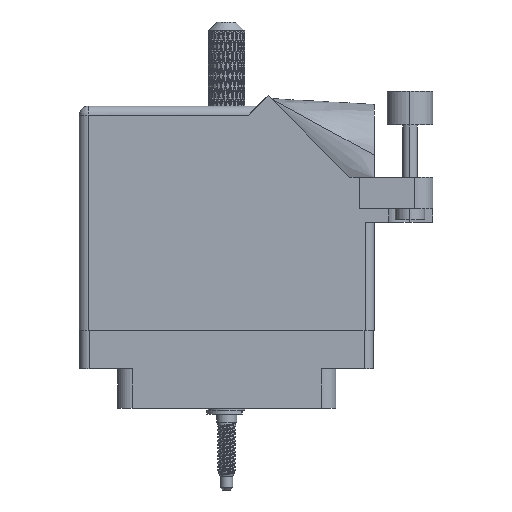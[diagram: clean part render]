
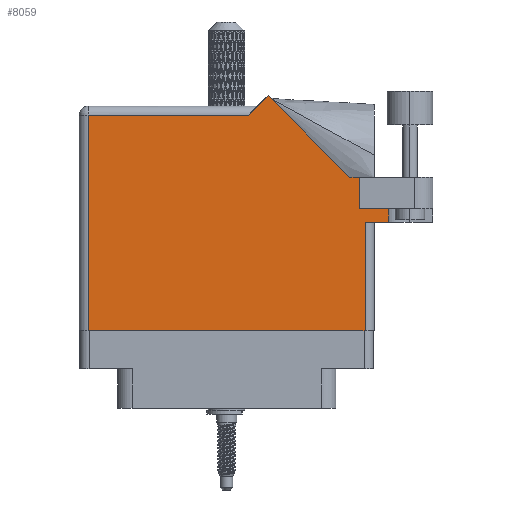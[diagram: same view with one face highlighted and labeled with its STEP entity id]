
A CAD part, front view. The second image highlights one B-rep face of the part: STEP entity #8059.
In plain terms, the highlighted face is planar.
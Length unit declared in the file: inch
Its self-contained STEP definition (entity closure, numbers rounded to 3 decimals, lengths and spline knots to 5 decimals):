
#267 = ORIENTED_EDGE ( 'NONE', *, *, #21707, .T. ) ;
#1807 = VECTOR ( 'NONE', #85075, 39.37008 ) ;
#2405 = VECTOR ( 'NONE', #69636, 39.37008 ) ;
#3095 = LINE ( 'NONE', #85515, #6949 ) ;
#5131 = CARTESIAN_POINT ( 'NONE',  ( 1.91, 0.831, 0. ) ) ;
#5653 = LINE ( 'NONE', #69418, #1807 ) ;
#6949 = VECTOR ( 'NONE', #50092, 39.37008 ) ;
#8059 = ADVANCED_FACE ( 'NONE', ( #53027 ), #77841, .F. ) ;
#8136 = DIRECTION ( 'NONE',  ( -1., 0., 0. ) ) ;
#8441 = DIRECTION ( 'NONE',  ( 0., 1., 0. ) ) ;
#9193 = LINE ( 'NONE', #20902, #78951 ) ;
#15080 = VERTEX_POINT ( 'NONE', #63916 ) ;
#15807 = CARTESIAN_POINT ( 'NONE',  ( 1.91, 0.831, 0. ) ) ;
#18346 = VERTEX_POINT ( 'NONE', #102619 ) ;
#19909 = VECTOR ( 'NONE', #8136, 39.37008 ) ;
#20902 = CARTESIAN_POINT ( 'NONE',  ( 0.062, 0., 0. ) ) ;
#21707 = EDGE_CURVE ( 'NONE', #97203, #96389, #76331, .T. ) ;
#24093 = CARTESIAN_POINT ( 'NONE',  ( 0., 1.468, 0. ) ) ;
#25519 = CARTESIAN_POINT ( 'NONE',  ( 2.1115, 0.737, 0. ) ) ;
#25620 = LINE ( 'NONE', #51140, #97981 ) ;
#27400 = EDGE_CURVE ( 'NONE', #18346, #99233, #84710, .T. ) ;
#27518 = EDGE_LOOP ( 'NONE', ( #94207, #48665, #95513, #96417, #34351, #267, #37238, #93862, #74592, #65399, #103088 ) ) ;
#27914 = AXIS2_PLACEMENT_3D ( 'NONE', #68934, #44972, #101667 ) ;
#28590 = CARTESIAN_POINT ( 'NONE',  ( 0.062, 0., 0. ) ) ;
#29988 = DIRECTION ( 'NONE',  ( 1., 0., 0. ) ) ;
#31210 = DIRECTION ( 'NONE',  ( 1., 0., 0. ) ) ;
#33255 = DIRECTION ( 'NONE',  ( -0.707, 0.707, 0. ) ) ;
#33606 = VERTEX_POINT ( 'NONE', #64223 ) ;
#34351 = ORIENTED_EDGE ( 'NONE', *, *, #74058, .F. ) ;
#37238 = ORIENTED_EDGE ( 'NONE', *, *, #104249, .T. ) ;
#38923 = LINE ( 'NONE', #98473, #65390 ) ;
#39635 = DIRECTION ( 'NONE',  ( 0., 1., 0. ) ) ;
#40151 = VECTOR ( 'NONE', #31210, 39.37008 ) ;
#41681 = VERTEX_POINT ( 'NONE', #93233 ) ;
#43035 = DIRECTION ( 'NONE',  ( 1., 0., 0. ) ) ;
#44609 = CARTESIAN_POINT ( 'NONE',  ( 2.1115, 0.831, 0. ) ) ;
#44972 = DIRECTION ( 'NONE',  ( 0., 0., -1. ) ) ;
#45186 = EDGE_CURVE ( 'NONE', #15080, #100135, #9193, .T. ) ;
#48665 = ORIENTED_EDGE ( 'NONE', *, *, #88799, .T. ) ;
#50092 = DIRECTION ( 'NONE',  ( -1., 0., 0. ) ) ;
#51140 = CARTESIAN_POINT ( 'NONE',  ( 2.01, 0.737, 0. ) ) ;
#53027 = FACE_OUTER_BOUND ( 'NONE', #27518, .T. ) ;
#53054 = EDGE_CURVE ( 'NONE', #41681, #79997, #25620, .T. ) ;
#53318 = CARTESIAN_POINT ( 'NONE',  ( 0., 0., 0. ) ) ;
#56301 = CARTESIAN_POINT ( 'NONE',  ( 1.948, 0.737, 0. ) ) ;
#57269 = VERTEX_POINT ( 'NONE', #44609 ) ;
#61670 = LINE ( 'NONE', #104939, #40151 ) ;
#61741 = EDGE_CURVE ( 'NONE', #100135, #33606, #100624, .T. ) ;
#63916 = CARTESIAN_POINT ( 'NONE',  ( 0.062, 1.468, 0. ) ) ;
#64223 = CARTESIAN_POINT ( 'NONE',  ( 1.948, 0., 0. ) ) ;
#65000 = VECTOR ( 'NONE', #39635, 39.37008 ) ;
#65390 = VECTOR ( 'NONE', #33255, 39.37008 ) ;
#65399 = ORIENTED_EDGE ( 'NONE', *, *, #86586, .T. ) ;
#68362 = DIRECTION ( 'NONE',  ( 0., -1., 0. ) ) ;
#68934 = CARTESIAN_POINT ( 'NONE',  ( 0., 1.53, 0. ) ) ;
#69418 = CARTESIAN_POINT ( 'NONE',  ( 2.1115, 1.16177, 0. ) ) ;
#69636 = DIRECTION ( 'NONE',  ( -0.707, -0.707, 0. ) ) ;
#71382 = VECTOR ( 'NONE', #29988, 39.37008 ) ;
#74058 = EDGE_CURVE ( 'NONE', #97203, #57269, #61670, .T. ) ;
#74206 = VECTOR ( 'NONE', #8441, 39.37008 ) ;
#74592 = ORIENTED_EDGE ( 'NONE', *, *, #27400, .T. ) ;
#76331 = LINE ( 'NONE', #15807, #65000 ) ;
#77841 = PLANE ( 'NONE',  #27914 ) ;
#78912 = CARTESIAN_POINT ( 'NONE',  ( 1.217, 1.53, 0. ) ) ;
#78951 = VECTOR ( 'NONE', #68362, 39.37008 ) ;
#79997 = VERTEX_POINT ( 'NONE', #25519 ) ;
#82376 = VERTEX_POINT ( 'NONE', #104918 ) ;
#84430 = LINE ( 'NONE', #56301, #74206 ) ;
#84710 = LINE ( 'NONE', #78912, #2405 ) ;
#85075 = DIRECTION ( 'NONE',  ( 0., -1., 0. ) ) ;
#85515 = CARTESIAN_POINT ( 'NONE',  ( 2.41, 1.044, 0. ) ) ;
#86586 = EDGE_CURVE ( 'NONE', #99233, #15080, #96104, .T. ) ;
#88799 = EDGE_CURVE ( 'NONE', #33606, #41681, #84430, .T. ) ;
#92310 = EDGE_CURVE ( 'NONE', #82376, #18346, #38923, .T. ) ;
#93233 = CARTESIAN_POINT ( 'NONE',  ( 1.948, 0.737, 0. ) ) ;
#93862 = ORIENTED_EDGE ( 'NONE', *, *, #92310, .T. ) ;
#94207 = ORIENTED_EDGE ( 'NONE', *, *, #61741, .T. ) ;
#95513 = ORIENTED_EDGE ( 'NONE', *, *, #53054, .T. ) ;
#96104 = LINE ( 'NONE', #24093, #19909 ) ;
#96389 = VERTEX_POINT ( 'NONE', #104495 ) ;
#96417 = ORIENTED_EDGE ( 'NONE', *, *, #97811, .F. ) ;
#97203 = VERTEX_POINT ( 'NONE', #5131 ) ;
#97811 = EDGE_CURVE ( 'NONE', #57269, #79997, #5653, .T. ) ;
#97981 = VECTOR ( 'NONE', #43035, 39.37008 ) ;
#98473 = CARTESIAN_POINT ( 'NONE',  ( 1.84442, 1.044, 0. ) ) ;
#99233 = VERTEX_POINT ( 'NONE', #103302 ) ;
#100135 = VERTEX_POINT ( 'NONE', #28590 ) ;
#100624 = LINE ( 'NONE', #53318, #71382 ) ;
#101667 = DIRECTION ( 'NONE',  ( -1., 0., 0. ) ) ;
#102619 = CARTESIAN_POINT ( 'NONE',  ( 1.28771, 1.60071, 0. ) ) ;
#103088 = ORIENTED_EDGE ( 'NONE', *, *, #45186, .T. ) ;
#103302 = CARTESIAN_POINT ( 'NONE',  ( 1.155, 1.468, 0. ) ) ;
#104249 = EDGE_CURVE ( 'NONE', #96389, #82376, #3095, .T. ) ;
#104495 = CARTESIAN_POINT ( 'NONE',  ( 1.91, 1.044, 0. ) ) ;
#104918 = CARTESIAN_POINT ( 'NONE',  ( 1.84442, 1.044, 0. ) ) ;
#104939 = CARTESIAN_POINT ( 'NONE',  ( 1.91, 0.831, 0. ) ) ;
